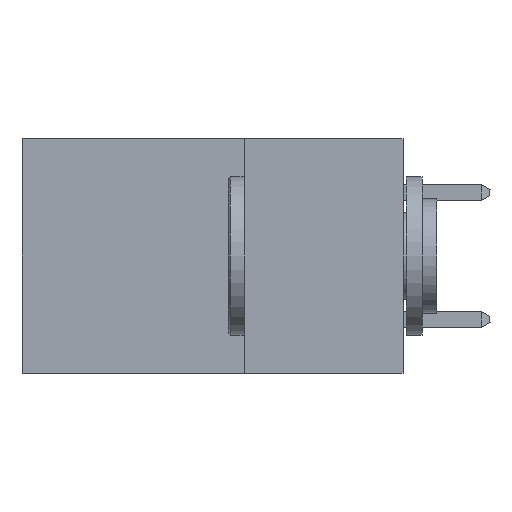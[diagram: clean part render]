
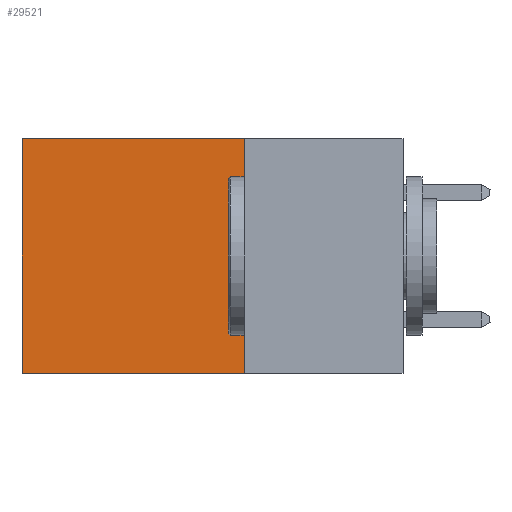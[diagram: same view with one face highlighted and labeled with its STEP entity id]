
A CAD part, left-side view. The second image highlights one B-rep face of the part: STEP entity #29521.
In plain terms, the highlighted planar face has unit normal (-1, 0, 0).
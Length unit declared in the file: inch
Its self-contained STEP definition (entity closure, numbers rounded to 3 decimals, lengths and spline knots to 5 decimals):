
#1503 = ORIENTED_EDGE ( 'NONE', *, *, #30622, .T. ) ;
#1819 = CARTESIAN_POINT ( 'NONE',  ( 0.2875, 0.6, 0. ) ) ;
#2355 = ORIENTED_EDGE ( 'NONE', *, *, #32607, .F. ) ;
#2516 = CARTESIAN_POINT ( 'NONE',  ( 0.2875, 0.25, -0.37 ) ) ;
#3417 = EDGE_CURVE ( 'NONE', #20185, #21006, #11023, .T. ) ;
#3443 = VECTOR ( 'NONE', #13361, 39.37008 ) ;
#4173 = CARTESIAN_POINT ( 'NONE',  ( 0.2875, 0.25, -0.37 ) ) ;
#5704 = VECTOR ( 'NONE', #24078, 39.37008 ) ;
#6631 = DIRECTION ( 'NONE',  ( 0., 0., -1. ) ) ;
#7506 = DIRECTION ( 'NONE',  ( 0., 0., -1. ) ) ;
#8266 = LINE ( 'NONE', #24552, #34124 ) ;
#8269 = EDGE_LOOP ( 'NONE', ( #1503, #2355, #11842, #33551 ) ) ;
#11023 = LINE ( 'NONE', #18729, #3443 ) ;
#11358 = VERTEX_POINT ( 'NONE', #4173 ) ;
#11842 = ORIENTED_EDGE ( 'NONE', *, *, #29039, .F. ) ;
#11882 = CARTESIAN_POINT ( 'NONE',  ( 0.2875, 0.25, 0. ) ) ;
#13361 = DIRECTION ( 'NONE',  ( 0., 1., 0. ) ) ;
#13474 = AXIS2_PLACEMENT_3D ( 'NONE', #20808, #29440, #6631 ) ;
#14121 = FACE_OUTER_BOUND ( 'NONE', #8269, .T. ) ;
#14711 = PLANE ( 'NONE',  #13474 ) ;
#18729 = CARTESIAN_POINT ( 'NONE',  ( 0.2875, 0.25, 0. ) ) ;
#19940 = LINE ( 'NONE', #20839, #5704 ) ;
#20185 = VERTEX_POINT ( 'NONE', #11882 ) ;
#20808 = CARTESIAN_POINT ( 'NONE',  ( 0.2875, 0.25, 0. ) ) ;
#20839 = CARTESIAN_POINT ( 'NONE',  ( 0.2875, 0.25, 0. ) ) ;
#21006 = VERTEX_POINT ( 'NONE', #1819 ) ;
#21402 = VECTOR ( 'NONE', #33984, 39.37008 ) ;
#24078 = DIRECTION ( 'NONE',  ( 0., 0., -1. ) ) ;
#24552 = CARTESIAN_POINT ( 'NONE',  ( 0.2875, 0.6, 0. ) ) ;
#29039 = EDGE_CURVE ( 'NONE', #20185, #11358, #19940, .T. ) ;
#29440 = DIRECTION ( 'NONE',  ( 1., 0., 0. ) ) ;
#29521 = ADVANCED_FACE ( 'NONE', ( #14121 ), #14711, .F. ) ;
#30355 = LINE ( 'NONE', #2516, #21402 ) ;
#30622 = EDGE_CURVE ( 'NONE', #21006, #31276, #8266, .T. ) ;
#31276 = VERTEX_POINT ( 'NONE', #34020 ) ;
#32607 = EDGE_CURVE ( 'NONE', #11358, #31276, #30355, .T. ) ;
#33551 = ORIENTED_EDGE ( 'NONE', *, *, #3417, .T. ) ;
#33984 = DIRECTION ( 'NONE',  ( 0., 1., 0. ) ) ;
#34020 = CARTESIAN_POINT ( 'NONE',  ( 0.2875, 0.6, -0.37 ) ) ;
#34124 = VECTOR ( 'NONE', #7506, 39.37008 ) ;
